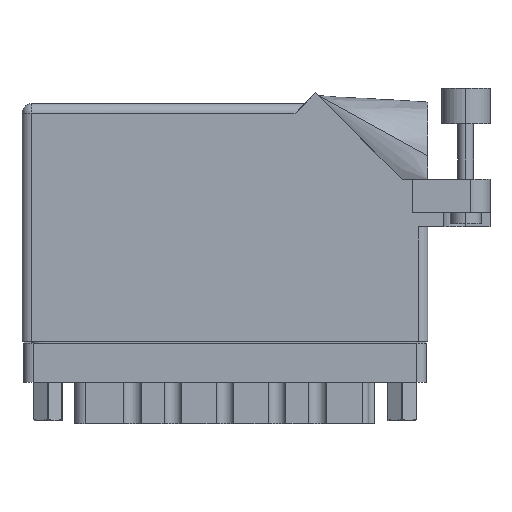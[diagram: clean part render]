
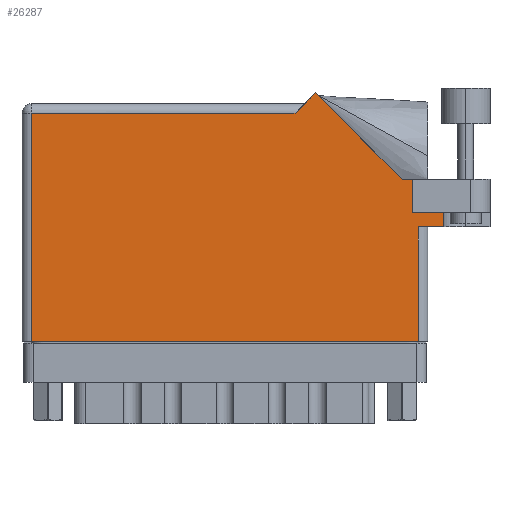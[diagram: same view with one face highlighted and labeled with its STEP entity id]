
A CAD part, front view. The second image highlights one B-rep face of the part: STEP entity #26287.
In plain terms, the highlighted face is planar.
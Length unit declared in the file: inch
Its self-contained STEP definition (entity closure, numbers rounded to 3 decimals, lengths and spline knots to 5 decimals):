
#648 = CARTESIAN_POINT ( 'NONE',  ( 2.44642, 1.044, 0. ) ) ;
#1756 = EDGE_CURVE ( 'NONE', #60353, #6348, #51923, .T. ) ;
#2356 = VERTEX_POINT ( 'NONE', #15113 ) ;
#2410 = CARTESIAN_POINT ( 'NONE',  ( 2.55, 0.737, 0. ) ) ;
#3145 = DIRECTION ( 'NONE',  ( 1., 0., 0. ) ) ;
#3246 = CARTESIAN_POINT ( 'NONE',  ( 3.012, 1.044, 0. ) ) ;
#3530 = EDGE_CURVE ( 'NONE', #6348, #37516, #13921, .T. ) ;
#4659 = VERTEX_POINT ( 'NONE', #24344 ) ;
#5075 = LINE ( 'NONE', #17452, #20896 ) ;
#5104 = VECTOR ( 'NONE', #12550, 39.37008 ) ;
#5301 = CARTESIAN_POINT ( 'NONE',  ( 0., 1.468, 0. ) ) ;
#5308 = CARTESIAN_POINT ( 'NONE',  ( 1.88971, 1.60071, 0. ) ) ;
#6006 = CARTESIAN_POINT ( 'NONE',  ( 0.062, 0., 0. ) ) ;
#6246 = DIRECTION ( 'NONE',  ( 1., 0., 0. ) ) ;
#6348 = VERTEX_POINT ( 'NONE', #648 ) ;
#6460 = CARTESIAN_POINT ( 'NONE',  ( 2.512, 0.831, 0. ) ) ;
#8069 = VERTEX_POINT ( 'NONE', #62148 ) ;
#11941 = LINE ( 'NONE', #5301, #60337 ) ;
#12509 = DIRECTION ( 'NONE',  ( 0., 0., -1. ) ) ;
#12550 = DIRECTION ( 'NONE',  ( 0., 1., 0. ) ) ;
#13134 = DIRECTION ( 'NONE',  ( -1., 0., 0. ) ) ;
#13279 = LINE ( 'NONE', #16404, #55633 ) ;
#13921 = LINE ( 'NONE', #29861, #57066 ) ;
#15113 = CARTESIAN_POINT ( 'NONE',  ( 0.062, 1.468, 0. ) ) ;
#16378 = ORIENTED_EDGE ( 'NONE', *, *, #43891, .T. ) ;
#16404 = CARTESIAN_POINT ( 'NONE',  ( 2.7135, 1.16177, 0. ) ) ;
#17452 = CARTESIAN_POINT ( 'NONE',  ( 2.612, 0.737, 0. ) ) ;
#17839 = EDGE_CURVE ( 'NONE', #36592, #57273, #53620, .T. ) ;
#18226 = LINE ( 'NONE', #20516, #50764 ) ;
#19200 = CARTESIAN_POINT ( 'NONE',  ( 2.7135, 0.831, 0. ) ) ;
#20149 = ORIENTED_EDGE ( 'NONE', *, *, #37713, .T. ) ;
#20516 = CARTESIAN_POINT ( 'NONE',  ( 0., 0., 0. ) ) ;
#20896 = VECTOR ( 'NONE', #3145, 39.37008 ) ;
#21259 = LINE ( 'NONE', #6006, #40200 ) ;
#21341 = EDGE_CURVE ( 'NONE', #57273, #31025, #13279, .T. ) ;
#23348 = AXIS2_PLACEMENT_3D ( 'NONE', #60919, #12509, #46333 ) ;
#24344 = CARTESIAN_POINT ( 'NONE',  ( 1.757, 1.468, 0. ) ) ;
#25489 = VERTEX_POINT ( 'NONE', #34699 ) ;
#26120 = CARTESIAN_POINT ( 'NONE',  ( 0.062, 0., 0. ) ) ;
#26287 = ADVANCED_FACE ( 'NONE', ( #56630 ), #51762, .F. ) ;
#26993 = EDGE_CURVE ( 'NONE', #25489, #31025, #5075, .T. ) ;
#27728 = LINE ( 'NONE', #2410, #5104 ) ;
#29095 = VERTEX_POINT ( 'NONE', #26120 ) ;
#29861 = CARTESIAN_POINT ( 'NONE',  ( 2.44642, 1.044, 0. ) ) ;
#30708 = EDGE_CURVE ( 'NONE', #4659, #2356, #11941, .T. ) ;
#30875 = ORIENTED_EDGE ( 'NONE', *, *, #1756, .T. ) ;
#31025 = VERTEX_POINT ( 'NONE', #44311 ) ;
#31649 = EDGE_LOOP ( 'NONE', ( #51214, #16378, #57005, #34682, #33017, #53442, #30875, #48479, #20149, #35228, #54698 ) ) ;
#33017 = ORIENTED_EDGE ( 'NONE', *, *, #17839, .F. ) ;
#34682 = ORIENTED_EDGE ( 'NONE', *, *, #21341, .F. ) ;
#34699 = CARTESIAN_POINT ( 'NONE',  ( 2.55, 0.737, 0. ) ) ;
#35037 = DIRECTION ( 'NONE',  ( -1., 0., 0. ) ) ;
#35228 = ORIENTED_EDGE ( 'NONE', *, *, #30708, .T. ) ;
#35750 = DIRECTION ( 'NONE',  ( 1., 0., 0. ) ) ;
#36103 = DIRECTION ( 'NONE',  ( -0.707, -0.707, 0. ) ) ;
#36592 = VERTEX_POINT ( 'NONE', #61836 ) ;
#37516 = VERTEX_POINT ( 'NONE', #5308 ) ;
#37713 = EDGE_CURVE ( 'NONE', #37516, #4659, #39105, .T. ) ;
#38457 = CARTESIAN_POINT ( 'NONE',  ( 2.512, 1.044, 0. ) ) ;
#39105 = LINE ( 'NONE', #50893, #46713 ) ;
#40200 = VECTOR ( 'NONE', #44658, 39.37008 ) ;
#42910 = DIRECTION ( 'NONE',  ( 0., 1., 0. ) ) ;
#43891 = EDGE_CURVE ( 'NONE', #8069, #25489, #27728, .T. ) ;
#44311 = CARTESIAN_POINT ( 'NONE',  ( 2.7135, 0.737, 0. ) ) ;
#44658 = DIRECTION ( 'NONE',  ( 0., -1., 0. ) ) ;
#44838 = VECTOR ( 'NONE', #42910, 39.37008 ) ;
#46333 = DIRECTION ( 'NONE',  ( -1., 0., 0. ) ) ;
#46713 = VECTOR ( 'NONE', #36103, 39.37008 ) ;
#48152 = VECTOR ( 'NONE', #13134, 39.37008 ) ;
#48479 = ORIENTED_EDGE ( 'NONE', *, *, #3530, .T. ) ;
#48946 = DIRECTION ( 'NONE',  ( -0.707, 0.707, 0. ) ) ;
#50764 = VECTOR ( 'NONE', #35750, 39.37008 ) ;
#50893 = CARTESIAN_POINT ( 'NONE',  ( 1.819, 1.53, 0. ) ) ;
#51214 = ORIENTED_EDGE ( 'NONE', *, *, #61810, .T. ) ;
#51762 = PLANE ( 'NONE',  #23348 ) ;
#51769 = CARTESIAN_POINT ( 'NONE',  ( 2.512, 0.831, 0. ) ) ;
#51923 = LINE ( 'NONE', #3246, #48152 ) ;
#53442 = ORIENTED_EDGE ( 'NONE', *, *, #57132, .T. ) ;
#53620 = LINE ( 'NONE', #6460, #56691 ) ;
#54698 = ORIENTED_EDGE ( 'NONE', *, *, #61872, .T. ) ;
#55633 = VECTOR ( 'NONE', #60183, 39.37008 ) ;
#56630 = FACE_OUTER_BOUND ( 'NONE', #31649, .T. ) ;
#56691 = VECTOR ( 'NONE', #6246, 39.37008 ) ;
#57005 = ORIENTED_EDGE ( 'NONE', *, *, #26993, .T. ) ;
#57066 = VECTOR ( 'NONE', #48946, 39.37008 ) ;
#57132 = EDGE_CURVE ( 'NONE', #36592, #60353, #60756, .T. ) ;
#57273 = VERTEX_POINT ( 'NONE', #19200 ) ;
#60183 = DIRECTION ( 'NONE',  ( 0., -1., 0. ) ) ;
#60337 = VECTOR ( 'NONE', #35037, 39.37008 ) ;
#60353 = VERTEX_POINT ( 'NONE', #38457 ) ;
#60756 = LINE ( 'NONE', #51769, #44838 ) ;
#60919 = CARTESIAN_POINT ( 'NONE',  ( 0., 1.53, 0. ) ) ;
#61810 = EDGE_CURVE ( 'NONE', #29095, #8069, #18226, .T. ) ;
#61836 = CARTESIAN_POINT ( 'NONE',  ( 2.512, 0.831, 0. ) ) ;
#61872 = EDGE_CURVE ( 'NONE', #2356, #29095, #21259, .T. ) ;
#62148 = CARTESIAN_POINT ( 'NONE',  ( 2.55, 0., 0. ) ) ;
